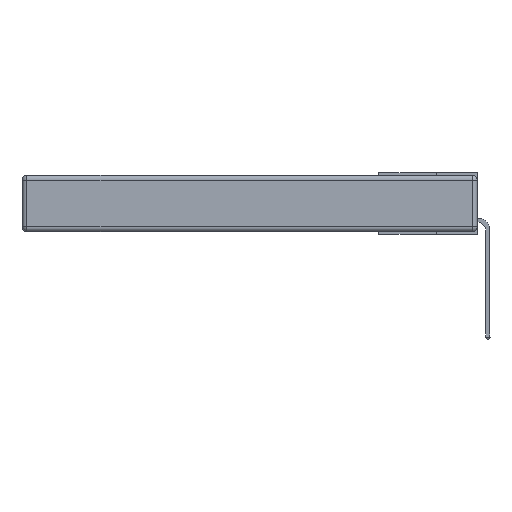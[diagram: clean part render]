
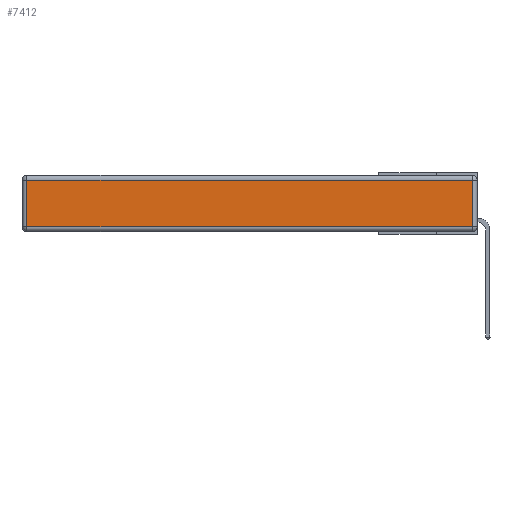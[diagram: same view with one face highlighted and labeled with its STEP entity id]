
A CAD part, left-side view. The second image highlights one B-rep face of the part: STEP entity #7412.
In plain terms, the highlighted planar face has unit normal (-1, 0, 0).
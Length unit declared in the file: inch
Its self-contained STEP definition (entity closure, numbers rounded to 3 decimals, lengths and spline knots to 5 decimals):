
#384 = AXIS2_PLACEMENT_3D ( 'NONE', #18265, #14145, #9939 ) ;
#1233 = LINE ( 'NONE', #12247, #1541 ) ;
#1541 = VECTOR ( 'NONE', #25089, 39.37008 ) ;
#2035 = EDGE_CURVE ( 'NONE', #10475, #13084, #1233, .T. ) ;
#3271 = PLANE ( 'NONE',  #384 ) ;
#3536 = CARTESIAN_POINT ( 'NONE',  ( 0., 2.75, -0.03 ) ) ;
#5364 = ORIENTED_EDGE ( 'NONE', *, *, #11581, .T. ) ;
#5689 = DIRECTION ( 'NONE',  ( 0., 1., 0. ) ) ;
#6257 = VECTOR ( 'NONE', #8562, 39.37008 ) ;
#6622 = ORIENTED_EDGE ( 'NONE', *, *, #27209, .T. ) ;
#7412 = ADVANCED_FACE ( 'NONE', ( #22217 ), #3271, .T. ) ;
#7708 = CARTESIAN_POINT ( 'NONE',  ( 0., 2.72, -0.313 ) ) ;
#7979 = ORIENTED_EDGE ( 'NONE', *, *, #2035, .T. ) ;
#8562 = DIRECTION ( 'NONE',  ( 0., -1., 0. ) ) ;
#8684 = ORIENTED_EDGE ( 'NONE', *, *, #17872, .T. ) ;
#9939 = DIRECTION ( 'NONE',  ( 0., 0., 1. ) ) ;
#10056 = DIRECTION ( 'NONE',  ( 0., 0., 1. ) ) ;
#10475 = VERTEX_POINT ( 'NONE', #21892 ) ;
#11581 = EDGE_CURVE ( 'NONE', #26533, #10475, #21768, .T. ) ;
#12247 = CARTESIAN_POINT ( 'NONE',  ( 0., 2.72, -0.343 ) ) ;
#12808 = CARTESIAN_POINT ( 'NONE',  ( 0., 0., -0.313 ) ) ;
#13084 = VERTEX_POINT ( 'NONE', #7708 ) ;
#14145 = DIRECTION ( 'NONE',  ( -1., 0., 0. ) ) ;
#16088 = LINE ( 'NONE', #12808, #6257 ) ;
#16353 = LINE ( 'NONE', #20455, #26891 ) ;
#17872 = EDGE_CURVE ( 'NONE', #13084, #23151, #16088, .T. ) ;
#18265 = CARTESIAN_POINT ( 'NONE',  ( 0., 0., -0.343 ) ) ;
#18869 = CARTESIAN_POINT ( 'NONE',  ( 0., 0.03, -0.313 ) ) ;
#20455 = CARTESIAN_POINT ( 'NONE',  ( 0., 0.03, -0.343 ) ) ;
#21612 = EDGE_LOOP ( 'NONE', ( #8684, #6622, #5364, #7979 ) ) ;
#21768 = LINE ( 'NONE', #3536, #23402 ) ;
#21892 = CARTESIAN_POINT ( 'NONE',  ( 0., 2.72, -0.03 ) ) ;
#22217 = FACE_OUTER_BOUND ( 'NONE', #21612, .T. ) ;
#23151 = VERTEX_POINT ( 'NONE', #18869 ) ;
#23402 = VECTOR ( 'NONE', #5689, 39.37008 ) ;
#23408 = CARTESIAN_POINT ( 'NONE',  ( 0., 0.03, -0.03 ) ) ;
#25089 = DIRECTION ( 'NONE',  ( 0., 0., -1. ) ) ;
#26533 = VERTEX_POINT ( 'NONE', #23408 ) ;
#26891 = VECTOR ( 'NONE', #10056, 39.37008 ) ;
#27209 = EDGE_CURVE ( 'NONE', #23151, #26533, #16353, .T. ) ;
